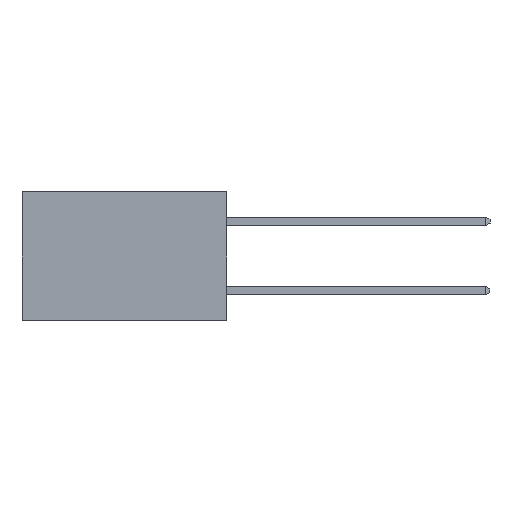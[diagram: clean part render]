
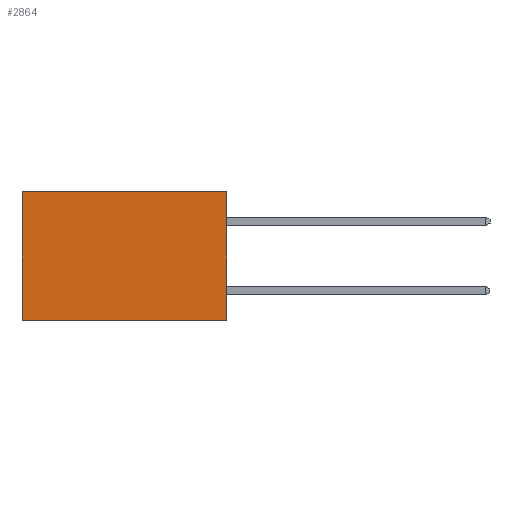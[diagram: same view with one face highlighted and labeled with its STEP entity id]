
A CAD part, left-side view. The second image highlights one B-rep face of the part: STEP entity #2864.
In plain terms, the highlighted planar face has unit normal (-1, 0, 0).
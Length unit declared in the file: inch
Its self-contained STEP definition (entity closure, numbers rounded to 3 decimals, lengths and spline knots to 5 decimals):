
#193 = DIRECTION ( 'NONE',  ( 0., 1., 0. ) ) ;
#529 = CARTESIAN_POINT ( 'NONE',  ( 0.277, 0.59, -0.37 ) ) ;
#1888 = LINE ( 'NONE', #2634, #25876 ) ;
#2405 = CARTESIAN_POINT ( 'NONE',  ( 0.277, 0., -0.37 ) ) ;
#2634 = CARTESIAN_POINT ( 'NONE',  ( 0.277, 0., 0. ) ) ;
#2699 = DIRECTION ( 'NONE',  ( 0., 0., -1. ) ) ;
#2768 = CARTESIAN_POINT ( 'NONE',  ( 0.277, 0., 0. ) ) ;
#2864 = ADVANCED_FACE ( 'NONE', ( #25588 ), #14336, .F. ) ;
#5665 = VECTOR ( 'NONE', #15039, 39.37008 ) ;
#6422 = LINE ( 'NONE', #17239, #18464 ) ;
#8054 = CARTESIAN_POINT ( 'NONE',  ( 0.277, 0.59, -0.37 ) ) ;
#8776 = ORIENTED_EDGE ( 'NONE', *, *, #13966, .F. ) ;
#10590 = LINE ( 'NONE', #529, #5665 ) ;
#11131 = CARTESIAN_POINT ( 'NONE',  ( 0.277, 0., -0.37 ) ) ;
#12311 = VERTEX_POINT ( 'NONE', #30713 ) ;
#13706 = EDGE_CURVE ( 'NONE', #20914, #18213, #1888, .T. ) ;
#13966 = EDGE_CURVE ( 'NONE', #12311, #16147, #6422, .T. ) ;
#14030 = EDGE_CURVE ( 'NONE', #18213, #16147, #10590, .T. ) ;
#14336 = PLANE ( 'NONE',  #28141 ) ;
#15039 = DIRECTION ( 'NONE',  ( 0., 0., -1. ) ) ;
#15955 = ORIENTED_EDGE ( 'NONE', *, *, #25017, .F. ) ;
#16147 = VERTEX_POINT ( 'NONE', #8054 ) ;
#16165 = DIRECTION ( 'NONE',  ( 1., 0., 0. ) ) ;
#16869 = DIRECTION ( 'NONE',  ( 0., 0., -1. ) ) ;
#17239 = CARTESIAN_POINT ( 'NONE',  ( 0.277, 0., -0.37 ) ) ;
#18198 = ORIENTED_EDGE ( 'NONE', *, *, #13706, .T. ) ;
#18213 = VERTEX_POINT ( 'NONE', #30555 ) ;
#18464 = VECTOR ( 'NONE', #22031, 39.37008 ) ;
#18546 = ORIENTED_EDGE ( 'NONE', *, *, #14030, .T. ) ;
#20597 = LINE ( 'NONE', #2405, #25359 ) ;
#20914 = VERTEX_POINT ( 'NONE', #2768 ) ;
#22031 = DIRECTION ( 'NONE',  ( 0., 1., 0. ) ) ;
#22186 = EDGE_LOOP ( 'NONE', ( #18546, #8776, #15955, #18198 ) ) ;
#25017 = EDGE_CURVE ( 'NONE', #20914, #12311, #20597, .T. ) ;
#25359 = VECTOR ( 'NONE', #16869, 39.37008 ) ;
#25588 = FACE_OUTER_BOUND ( 'NONE', #22186, .T. ) ;
#25876 = VECTOR ( 'NONE', #193, 39.37008 ) ;
#28141 = AXIS2_PLACEMENT_3D ( 'NONE', #11131, #16165, #2699 ) ;
#30555 = CARTESIAN_POINT ( 'NONE',  ( 0.277, 0.59, 0. ) ) ;
#30713 = CARTESIAN_POINT ( 'NONE',  ( 0.277, 0., -0.37 ) ) ;
